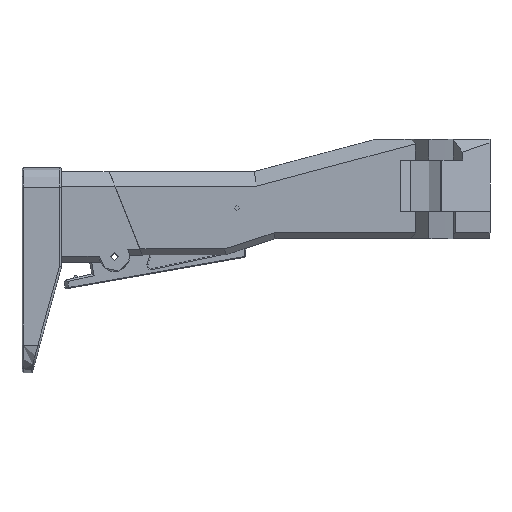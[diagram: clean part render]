
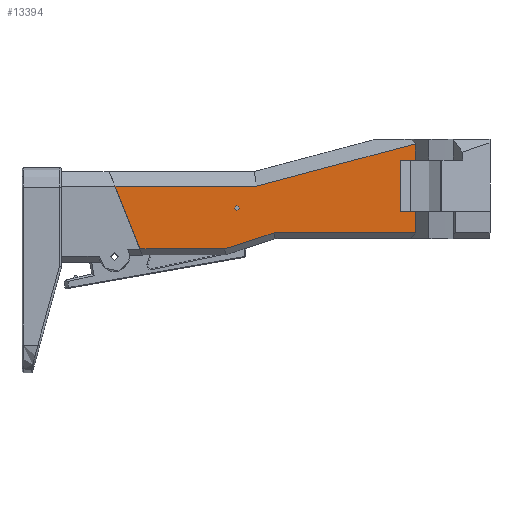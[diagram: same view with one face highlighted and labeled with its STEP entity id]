
A CAD part, top view. The second image highlights one B-rep face of the part: STEP entity #13394.
In plain terms, the highlighted planar face has unit normal (0, 0, 1).
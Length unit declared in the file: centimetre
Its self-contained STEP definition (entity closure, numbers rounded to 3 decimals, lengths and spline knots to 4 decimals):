
#198=FACE_BOUND($,#2049,.T.);
#515=PLANE($,#14440);
#1257=FACE_OUTER_BOUND($,#2048,.T.);
#2048=EDGE_LOOP($,(#11277,#11278,#11279,#11280,#11281,#11282,#11283,#11284,
#11285,#11286,#11287));
#2049=EDGE_LOOP($,(#11288));
#3240=LINE($,#21865,#4676);
#3287=LINE($,#21967,#4723);
#3288=LINE($,#21969,#4724);
#3289=LINE($,#21971,#4725);
#3290=LINE($,#21973,#4726);
#3291=LINE($,#21975,#4727);
#3292=LINE($,#21977,#4728);
#3293=LINE($,#21979,#4729);
#3294=LINE($,#21981,#4730);
#3295=LINE($,#21983,#4731);
#3296=LINE($,#21984,#4732);
#4676=VECTOR($,#17223,3.427);
#4723=VECTOR($,#17294,4.2997);
#4724=VECTOR($,#17295,2.631);
#4725=VECTOR($,#17296,7.1624);
#4726=VECTOR($,#17297,1.075);
#4727=VECTOR($,#17298,0.7375);
#4728=VECTOR($,#17299,2.61);
#4729=VECTOR($,#17300,0.7375);
#4730=VECTOR($,#17301,0.8238);
#4731=VECTOR($,#17302,8.3408);
#4732=VECTOR($,#17303,7.1665);
#5513=CIRCLE($,#14441,0.11);
#6409=VERTEX_POINT($,#21862);
#6410=VERTEX_POINT($,#21864);
#6453=VERTEX_POINT($,#21966);
#6454=VERTEX_POINT($,#21968);
#6455=VERTEX_POINT($,#21970);
#6456=VERTEX_POINT($,#21972);
#6457=VERTEX_POINT($,#21974);
#6458=VERTEX_POINT($,#21976);
#6459=VERTEX_POINT($,#21978);
#6460=VERTEX_POINT($,#21980);
#6461=VERTEX_POINT($,#21982);
#6462=VERTEX_POINT($,#21985);
#8090=EDGE_CURVE($,#6410,#6409,#3240,.T.);
#8141=EDGE_CURVE($,#6453,#6409,#3287,.T.);
#8142=EDGE_CURVE($,#6454,#6453,#3288,.T.);
#8143=EDGE_CURVE($,#6455,#6454,#3289,.T.);
#8144=EDGE_CURVE($,#6456,#6455,#3290,.T.);
#8145=EDGE_CURVE($,#6456,#6457,#3291,.T.);
#8146=EDGE_CURVE($,#6457,#6458,#3292,.T.);
#8147=EDGE_CURVE($,#6458,#6459,#3293,.T.);
#8148=EDGE_CURVE($,#6460,#6459,#3294,.T.);
#8149=EDGE_CURVE($,#6461,#6460,#3295,.T.);
#8150=EDGE_CURVE($,#6410,#6461,#3296,.T.);
#8151=EDGE_CURVE($,#6462,#6462,#5513,.T.);
#11277=ORIENTED_EDGE($,*,*,#8090,.T.);
#11278=ORIENTED_EDGE($,*,*,#8141,.F.);
#11279=ORIENTED_EDGE($,*,*,#8142,.F.);
#11280=ORIENTED_EDGE($,*,*,#8143,.F.);
#11281=ORIENTED_EDGE($,*,*,#8144,.F.);
#11282=ORIENTED_EDGE($,*,*,#8145,.T.);
#11283=ORIENTED_EDGE($,*,*,#8146,.T.);
#11284=ORIENTED_EDGE($,*,*,#8147,.T.);
#11285=ORIENTED_EDGE($,*,*,#8148,.F.);
#11286=ORIENTED_EDGE($,*,*,#8149,.F.);
#11287=ORIENTED_EDGE($,*,*,#8150,.F.);
#11288=ORIENTED_EDGE($,*,*,#8151,.T.);
#13394=ADVANCED_FACE($,(#1257,#198),#515,.T.);
#14440=AXIS2_PLACEMENT_3D($,#21965,#17292,#17293);
#14441=AXIS2_PLACEMENT_3D($,#21986,#17304,#17305);
#17223=DIRECTION($,(0.369,-0.929,0.));
#17292=DIRECTION('center_axis',(0.,0.,
1.));
#17293=DIRECTION('ref_axis',(1.,0.,0.));
#17294=DIRECTION($,(-1.,0.,0.));
#17295=DIRECTION($,(-0.95,-0.312,0.));
#17296=DIRECTION($,(-1.,0.,0.));
#17297=DIRECTION($,(0.,-1.,0.));
#17298=DIRECTION($,(-1.,0.,0.));
#17299=DIRECTION($,(0.,1.,0.));
#17300=DIRECTION($,(1.,0.,0.));
#17301=DIRECTION($,(0.,-1.,0.));
#17302=DIRECTION($,(0.966,0.257,0.));
#17303=DIRECTION($,(1.,0.,0.));
#17304=DIRECTION('center_axis',(0.,0.,
-1.));
#17305=DIRECTION('ref_axis',(-1.,0.,0.));
#21862=CARTESIAN_POINT('',(-37.549,-0.4636,11.6297));
#21864=CARTESIAN_POINT('',(-38.814,2.7214,11.6297));
#21865=CARTESIAN_POINT($,(-36.9099,-2.0727,11.6297));
#21965=CARTESIAN_POINT('Origin',(-21.7548,0.0564,11.6297));
#21966=CARTESIAN_POINT('',(-33.2492,-0.4636,11.6297));
#21967=CARTESIAN_POINT($,(-38.3748,-0.4636,11.6297));
#21968=CARTESIAN_POINT('',(-30.7492,0.3564,11.6297));
#21969=CARTESIAN_POINT($,(-26.7561,1.6661,11.6297));
#21970=CARTESIAN_POINT('',(-23.5869,0.3564,11.6297));
#21971=CARTESIAN_POINT($,(-21.7548,0.3564,11.6297));
#21972=CARTESIAN_POINT('',(-23.5869,1.4314,11.6297));
#21973=CARTESIAN_POINT($,(-23.5869,0.0564,11.6297));
#21974=CARTESIAN_POINT('',(-24.3244,1.4314,11.6297));
#21975=CARTESIAN_POINT($,(-20.0472,1.4314,11.6297));
#21976=CARTESIAN_POINT('',(-24.3244,4.0414,11.6297));
#21977=CARTESIAN_POINT($,(-24.3244,2.0489,11.6297));
#21978=CARTESIAN_POINT('',(-23.5869,4.0414,11.6297));
#21979=CARTESIAN_POINT($,(-20.0279,4.0414,11.6297));
#21980=CARTESIAN_POINT('',(-23.5869,4.8651,11.6297));
#21981=CARTESIAN_POINT($,(-23.5869,2.7314,11.6297));
#21982=CARTESIAN_POINT('',(-31.6474,2.7214,11.6297));
#21983=CARTESIAN_POINT($,(-27.3118,3.8744,11.6297));
#21984=CARTESIAN_POINT($,(-31.0048,2.7214,11.6297));
#21985=CARTESIAN_POINT('',(-32.5198,1.6114,11.6297));
#21986=CARTESIAN_POINT('Origin',(-32.6298,1.6114,11.6297));
